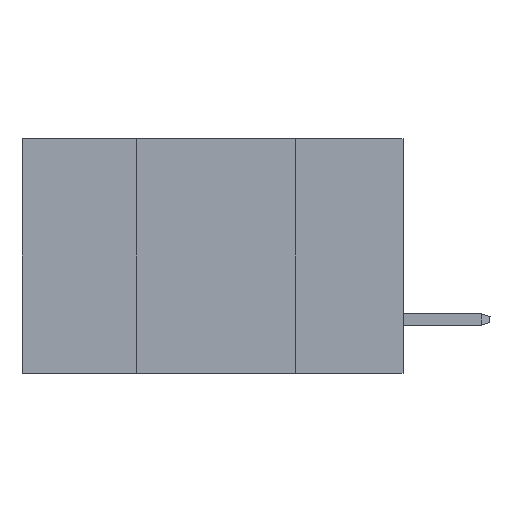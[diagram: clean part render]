
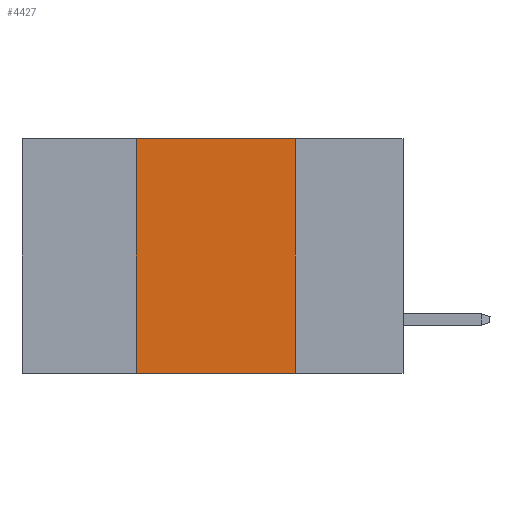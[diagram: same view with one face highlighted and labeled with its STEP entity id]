
A CAD part, left-side view. The second image highlights one B-rep face of the part: STEP entity #4427.
In plain terms, the highlighted planar face has unit normal (-1, 0, 0).
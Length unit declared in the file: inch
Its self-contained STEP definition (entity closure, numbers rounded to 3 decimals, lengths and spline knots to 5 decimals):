
#2013 = FACE_OUTER_BOUND ( 'NONE', #3441, .T. ) ;
#2303 = DIRECTION ( 'NONE',  ( 0., -1., 0. ) ) ;
#3441 = EDGE_LOOP ( 'NONE', ( #17503, #21668, #18012, #38137 ) ) ;
#3466 = CARTESIAN_POINT ( 'NONE',  ( 0., 0.17, 0. ) ) ;
#3833 = DIRECTION ( 'NONE',  ( 0., 0., 1. ) ) ;
#4427 = ADVANCED_FACE ( 'NONE', ( #2013 ), #36024, .F. ) ;
#6252 = EDGE_CURVE ( 'NONE', #20109, #27761, #12188, .T. ) ;
#7988 = VECTOR ( 'NONE', #2303, 39.37008 ) ;
#9734 = VERTEX_POINT ( 'NONE', #30068 ) ;
#10324 = CARTESIAN_POINT ( 'NONE',  ( 0., 0.17, -0.37 ) ) ;
#12188 = LINE ( 'NONE', #3466, #23854 ) ;
#13682 = CARTESIAN_POINT ( 'NONE',  ( 0., 0.42, 0. ) ) ;
#15566 = DIRECTION ( 'NONE',  ( 0., 0., -1. ) ) ;
#15800 = EDGE_CURVE ( 'NONE', #9734, #16309, #31095, .T. ) ;
#16309 = VERTEX_POINT ( 'NONE', #13682 ) ;
#17503 = ORIENTED_EDGE ( 'NONE', *, *, #6252, .F. ) ;
#17883 = DIRECTION ( 'NONE',  ( 1., 0., 0. ) ) ;
#18012 = ORIENTED_EDGE ( 'NONE', *, *, #15800, .F. ) ;
#18301 = DIRECTION ( 'NONE',  ( 0., 0., -1. ) ) ;
#18537 = CARTESIAN_POINT ( 'NONE',  ( 0., 0.17, 0. ) ) ;
#18542 = CARTESIAN_POINT ( 'NONE',  ( 0., 0.42, 0. ) ) ;
#19506 = EDGE_CURVE ( 'NONE', #9734, #27761, #38850, .T. ) ;
#20109 = VERTEX_POINT ( 'NONE', #18537 ) ;
#21668 = ORIENTED_EDGE ( 'NONE', *, *, #24831, .F. ) ;
#23854 = VECTOR ( 'NONE', #15566, 39.37008 ) ;
#24831 = EDGE_CURVE ( 'NONE', #16309, #20109, #25022, .T. ) ;
#25022 = LINE ( 'NONE', #25603, #33851 ) ;
#25603 = CARTESIAN_POINT ( 'NONE',  ( 0., 0.6, 0. ) ) ;
#26353 = VECTOR ( 'NONE', #3833, 39.37008 ) ;
#27761 = VERTEX_POINT ( 'NONE', #10324 ) ;
#28509 = AXIS2_PLACEMENT_3D ( 'NONE', #36206, #17883, #18301 ) ;
#28774 = DIRECTION ( 'NONE',  ( 0., -1., 0. ) ) ;
#30068 = CARTESIAN_POINT ( 'NONE',  ( 0., 0.42, -0.37 ) ) ;
#31095 = LINE ( 'NONE', #18542, #26353 ) ;
#33851 = VECTOR ( 'NONE', #28774, 39.37008 ) ;
#36024 = PLANE ( 'NONE',  #28509 ) ;
#36206 = CARTESIAN_POINT ( 'NONE',  ( 0., 0.6, 0. ) ) ;
#36298 = CARTESIAN_POINT ( 'NONE',  ( 0., 0.6, -0.37 ) ) ;
#38137 = ORIENTED_EDGE ( 'NONE', *, *, #19506, .T. ) ;
#38850 = LINE ( 'NONE', #36298, #7988 ) ;
